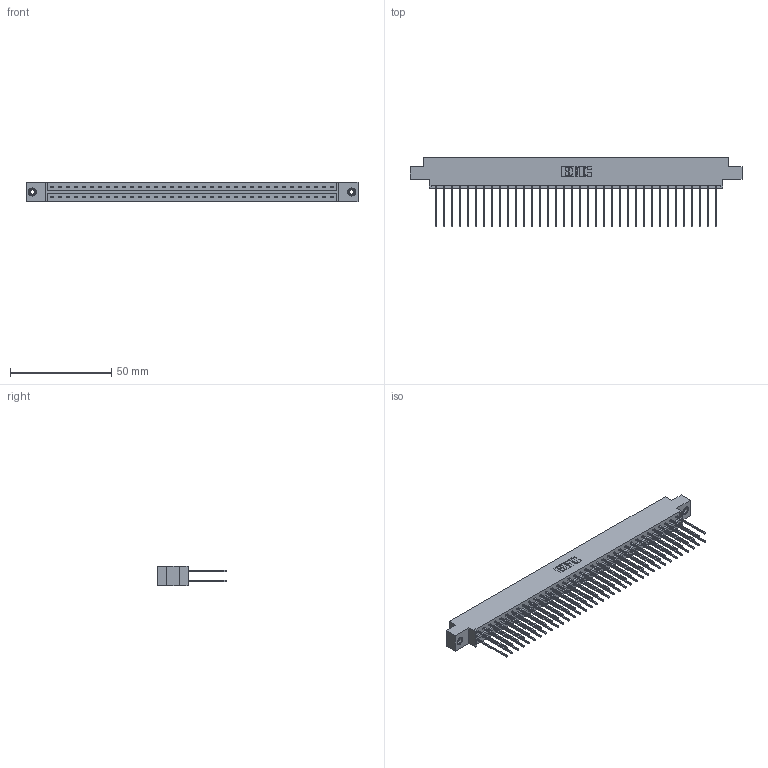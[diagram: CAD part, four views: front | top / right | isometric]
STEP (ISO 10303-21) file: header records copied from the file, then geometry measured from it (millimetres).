
FILE_DESCRIPTION (( 'STEP AP203' ), '1' );
FILE_NAME ('333-072-541-808.STEP', '2018-08-04T20:52:17', ( '' ), ( '' ), 'SwSTEP 2.0', 'SolidWorks 2016', '' );
FILE_SCHEMA (( 'CONFIG_CONTROL_DESIGN' ));
Length unit declared in the file: inch
Products named in the file (4): 333 Part_Offset - .156 Dia - TI; 345-292-001_345-293-141; 345-250-001_345-250-003-102; 333-072-541-808
Assembly tree (75 placements, depth 2):
  333-072-541-808
    333 Part_Offset - .156 Dia - TI
    345-292-001_345-293-141  x72
    345-250-001_345-250-003-102  x2
Bounding box: 164.19 x 34.3 x 9.4 mm (x, y, z)
Volume: 16885.1 mm3; surface area: 22197.3 mm2
Topology: 75 solids, 75 shells, 3922 faces, 11619 edges, 7642 vertices
Faces by surface type: plane 2698, cylinder 1208, cone 12, torus 4
Entity records: 25272 total; most frequent: CARTESIAN_POINT 4181, ORIENTED_EDGE 4110, DIRECTION 3613, EDGE_CURVE 2055, LINE 1907, VECTOR 1907, VERTEX_POINT 1364, AXIS2_PLACEMENT_3D 853
